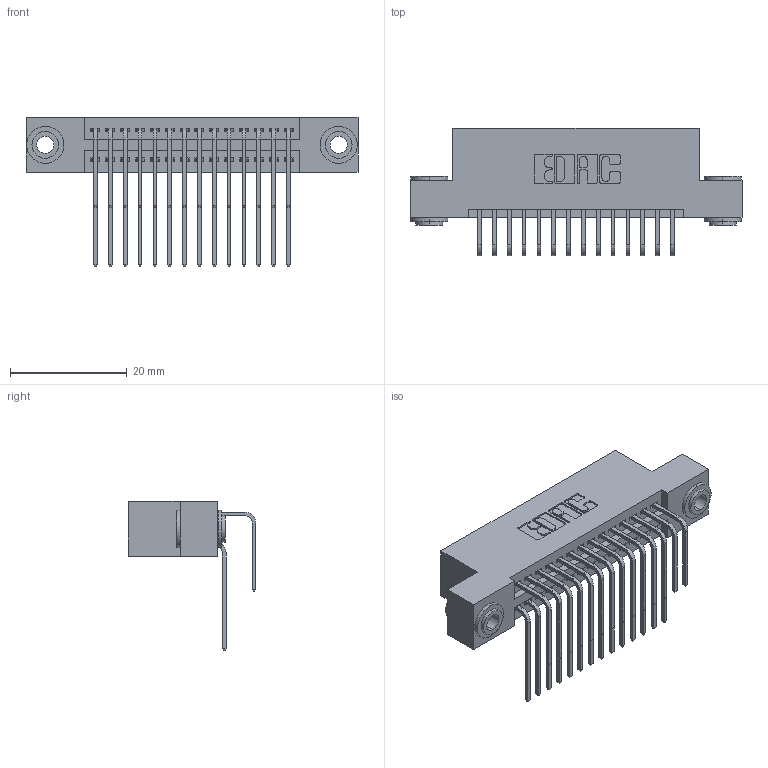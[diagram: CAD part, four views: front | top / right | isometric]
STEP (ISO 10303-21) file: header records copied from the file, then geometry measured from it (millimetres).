
FILE_DESCRIPTION (( 'STEP AP203' ), '1' );
FILE_NAME ('345-028-558-203.STEP', '2019-10-28T00:35:32', ( '' ), ( '' ), 'SwSTEP 2.0', 'SolidWorks 2016', '' );
FILE_SCHEMA (( 'CONFIG_CONTROL_DESIGN' ));
Length unit declared in the file: inch
Products named in the file (5): 345-292-001_558 Tail - 2; 345 Part_Flush Mounting Lugs - 0.156 Dia-TH; 345-028-558-203; 345-292-001_558 559 Tail - 1; 345-250-002_345-250-002-102
Assembly tree (31 placements, depth 2):
  345-028-558-203
    345 Part_Flush Mounting Lugs - 0.156 Dia-TH
    345-292-001_558 559 Tail - 1  x14
    345-292-001_558 Tail - 2  x14
    345-250-002_345-250-002-102  x2
Bounding box: 56.77 x 21.83 x 25.53 mm (x, y, z)
Volume: 5435.6 mm3; surface area: 8456.9 mm2
Topology: 31 solids, 31 shells, 1620 faces, 4757 edges, 3130 vertices
Faces by surface type: plane 1070, cylinder 542, cone 8
Entity records: 17056 total; most frequent: CARTESIAN_POINT 2906, ORIENTED_EDGE 2782, DIRECTION 2601, EDGE_CURVE 1391, LINE 1139, VECTOR 1139, VERTEX_POINT 922, AXIS2_PLACEMENT_3D 731
